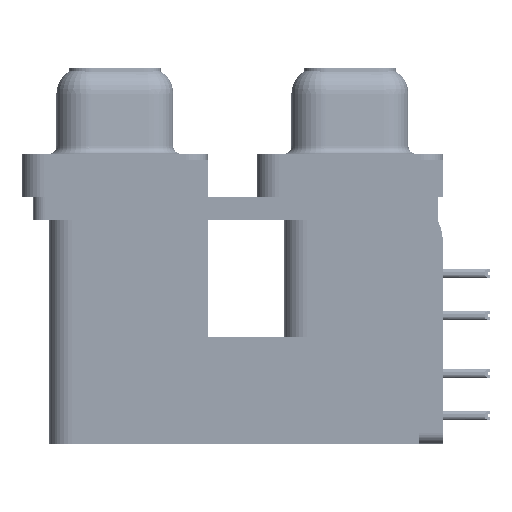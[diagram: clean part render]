
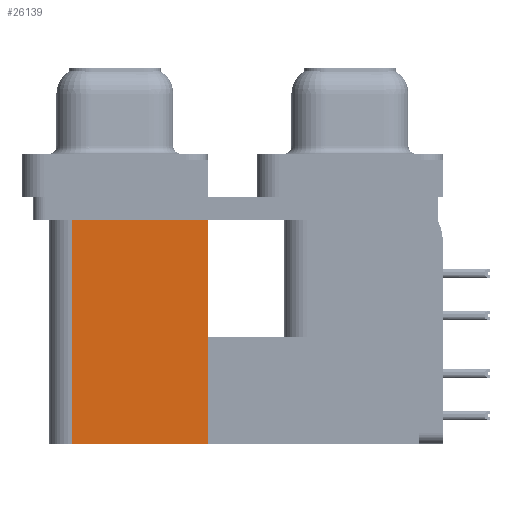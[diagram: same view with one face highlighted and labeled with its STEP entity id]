
A CAD part, left-side view. The second image highlights one B-rep face of the part: STEP entity #26139.
In plain terms, the highlighted planar face has unit normal (-1, 0, 0).
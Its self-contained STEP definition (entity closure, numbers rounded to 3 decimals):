
#994 = DIRECTION ( 'NONE',  ( 0., 1., 0. ) ) ;
#1021 = VERTEX_POINT ( 'NONE', #49109 ) ;
#4171 = LINE ( 'NONE', #55528, #38394 ) ;
#4541 = EDGE_CURVE ( 'NONE', #16343, #17630, #56099, .T. ) ;
#5069 = DIRECTION ( 'NONE',  ( 0., 1., 0. ) ) ;
#12539 = EDGE_CURVE ( 'NONE', #56618, #1021, #15393, .T. ) ;
#13667 = CARTESIAN_POINT ( 'NONE',  ( 3.7, 18.8, -2.5 ) ) ;
#14153 = ORIENTED_EDGE ( 'NONE', *, *, #48430, .F. ) ;
#14223 = DIRECTION ( 'NONE',  ( 0., 0., 1. ) ) ;
#15033 = ORIENTED_EDGE ( 'NONE', *, *, #12539, .T. ) ;
#15393 = LINE ( 'NONE', #52954, #53519 ) ;
#15995 = DIRECTION ( 'NONE',  ( 1., 0., 0. ) ) ;
#16343 = VERTEX_POINT ( 'NONE', #17737 ) ;
#17630 = VERTEX_POINT ( 'NONE', #13667 ) ;
#17737 = CARTESIAN_POINT ( 'NONE',  ( 3.7, 18.8, -19.2 ) ) ;
#21695 = CARTESIAN_POINT ( 'NONE',  ( 3.7, 9.6, -19.2 ) ) ;
#22529 = VECTOR ( 'NONE', #47523, 1000. ) ;
#24255 = FACE_OUTER_BOUND ( 'NONE', #38747, .T. ) ;
#25456 = DIRECTION ( 'NONE',  ( 0., 0., 1. ) ) ;
#25742 = EDGE_CURVE ( 'NONE', #1021, #17630, #4171, .T. ) ;
#26139 = ADVANCED_FACE ( 'NONE', ( #24255 ), #52949, .F. ) ;
#30419 = VECTOR ( 'NONE', #14223, 1000. ) ;
#33402 = ORIENTED_EDGE ( 'NONE', *, *, #25742, .T. ) ;
#38072 = CARTESIAN_POINT ( 'NONE',  ( 3.7, 9.6, -19.2 ) ) ;
#38377 = LINE ( 'NONE', #38072, #22529 ) ;
#38394 = VECTOR ( 'NONE', #5069, 1000. ) ;
#38747 = EDGE_LOOP ( 'NONE', ( #33402, #46328, #14153, #15033 ) ) ;
#46328 = ORIENTED_EDGE ( 'NONE', *, *, #4541, .F. ) ;
#46920 = CARTESIAN_POINT ( 'NONE',  ( 3.7, 18.8, -19.2 ) ) ;
#47523 = DIRECTION ( 'NONE',  ( 0., 1., 0. ) ) ;
#48073 = CARTESIAN_POINT ( 'NONE',  ( 3.7, 9.6, -19.2 ) ) ;
#48430 = EDGE_CURVE ( 'NONE', #56618, #16343, #38377, .T. ) ;
#49109 = CARTESIAN_POINT ( 'NONE',  ( 3.7, 9.6, -2.5 ) ) ;
#52103 = AXIS2_PLACEMENT_3D ( 'NONE', #48073, #15995, #994 ) ;
#52949 = PLANE ( 'NONE',  #52103 ) ;
#52954 = CARTESIAN_POINT ( 'NONE',  ( 3.7, 9.6, -19.2 ) ) ;
#53519 = VECTOR ( 'NONE', #25456, 1000. ) ;
#55528 = CARTESIAN_POINT ( 'NONE',  ( 3.7, 9.6, -2.5 ) ) ;
#56099 = LINE ( 'NONE', #46920, #30419 ) ;
#56618 = VERTEX_POINT ( 'NONE', #21695 ) ;
